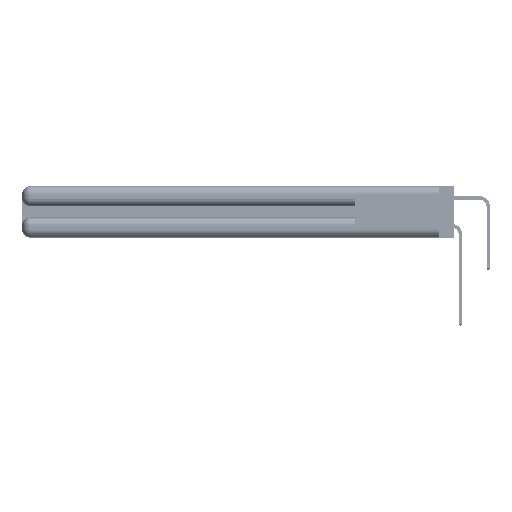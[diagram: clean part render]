
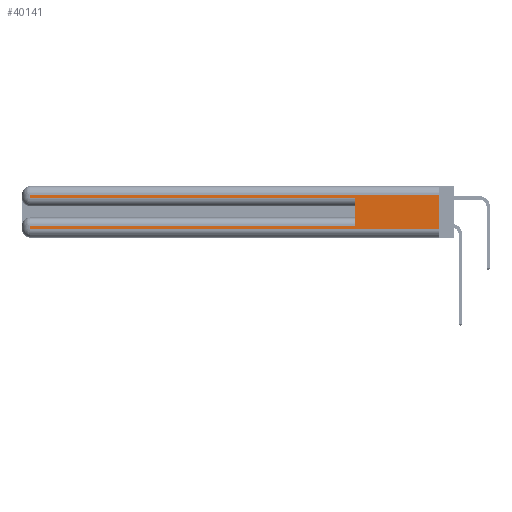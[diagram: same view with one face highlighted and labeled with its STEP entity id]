
A CAD part, left-side view. The second image highlights one B-rep face of the part: STEP entity #40141.
In plain terms, the highlighted planar face has unit normal (-1, 0, 0).
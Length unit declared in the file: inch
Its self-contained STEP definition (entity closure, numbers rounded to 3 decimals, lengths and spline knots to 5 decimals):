
#798 = VERTEX_POINT ( 'NONE', #17650 ) ;
#2021 = CARTESIAN_POINT ( 'NONE',  ( 0., 2.94, 0.06 ) ) ;
#2436 = ORIENTED_EDGE ( 'NONE', *, *, #35362, .T. ) ;
#2768 = CARTESIAN_POINT ( 'NONE',  ( 0., 2.94, 0.285 ) ) ;
#2984 = EDGE_CURVE ( 'NONE', #15669, #55443, #12551, .T. ) ;
#4035 = EDGE_CURVE ( 'NONE', #9120, #798, #41497, .T. ) ;
#4609 = CARTESIAN_POINT ( 'NONE',  ( 0., 2.94, 0.31 ) ) ;
#4824 = VERTEX_POINT ( 'NONE', #26628 ) ;
#4967 = ORIENTED_EDGE ( 'NONE', *, *, #2984, .F. ) ;
#5158 = CARTESIAN_POINT ( 'NONE',  ( 0., 0., 0.085 ) ) ;
#5236 = EDGE_CURVE ( 'NONE', #55634, #798, #55422, .T. ) ;
#5494 = LINE ( 'NONE', #29674, #10962 ) ;
#9120 = VERTEX_POINT ( 'NONE', #2021 ) ;
#10962 = VECTOR ( 'NONE', #12107, 39.37008 ) ;
#11747 = ORIENTED_EDGE ( 'NONE', *, *, #28604, .T. ) ;
#12107 = DIRECTION ( 'NONE',  ( 0., 1., 0. ) ) ;
#12335 = LINE ( 'NONE', #5158, #55706 ) ;
#12377 = DIRECTION ( 'NONE',  ( 1., 0., 0. ) ) ;
#12551 = LINE ( 'NONE', #27967, #22717 ) ;
#12958 = DIRECTION ( 'NONE',  ( 0., -1., 0. ) ) ;
#13211 = DIRECTION ( 'NONE',  ( 0., 0., -1. ) ) ;
#14215 = LINE ( 'NONE', #51944, #25746 ) ;
#14616 = CARTESIAN_POINT ( 'NONE',  ( 0., 0., 0.31 ) ) ;
#15669 = VERTEX_POINT ( 'NONE', #37559 ) ;
#16627 = FACE_OUTER_BOUND ( 'NONE', #29875, .T. ) ;
#16932 = CARTESIAN_POINT ( 'NONE',  ( 0., 0., 0.37 ) ) ;
#17650 = CARTESIAN_POINT ( 'NONE',  ( 0., 0., 0.06 ) ) ;
#20690 = CARTESIAN_POINT ( 'NONE',  ( 0., 0., 0.37 ) ) ;
#21822 = AXIS2_PLACEMENT_3D ( 'NONE', #16932, #12377, #33522 ) ;
#22451 = DIRECTION ( 'NONE',  ( 0., 1., 0. ) ) ;
#22717 = VECTOR ( 'NONE', #36632, 39.37008 ) ;
#23726 = CARTESIAN_POINT ( 'NONE',  ( 0., 0.6, 0.285 ) ) ;
#24527 = EDGE_CURVE ( 'NONE', #15669, #4824, #12335, .T. ) ;
#24696 = EDGE_CURVE ( 'NONE', #55634, #25555, #5494, .T. ) ;
#24818 = VECTOR ( 'NONE', #53105, 39.37008 ) ;
#25555 = VERTEX_POINT ( 'NONE', #4609 ) ;
#25746 = VECTOR ( 'NONE', #12958, 39.37008 ) ;
#26230 = ORIENTED_EDGE ( 'NONE', *, *, #5236, .F. ) ;
#26628 = CARTESIAN_POINT ( 'NONE',  ( 0., 2.94, 0.085 ) ) ;
#27967 = CARTESIAN_POINT ( 'NONE',  ( 0., 0.6, 0.145 ) ) ;
#28604 = EDGE_CURVE ( 'NONE', #25555, #34652, #41723, .T. ) ;
#28907 = VECTOR ( 'NONE', #13211, 39.37008 ) ;
#29674 = CARTESIAN_POINT ( 'NONE',  ( 0., 0., 0.31 ) ) ;
#29875 = EDGE_LOOP ( 'NONE', ( #26230, #30563, #11747, #2436, #4967, #53065, #35982, #38648 ) ) ;
#30563 = ORIENTED_EDGE ( 'NONE', *, *, #24696, .T. ) ;
#30599 = CARTESIAN_POINT ( 'NONE',  ( 0., 2.94, 0.37 ) ) ;
#31570 = EDGE_CURVE ( 'NONE', #4824, #9120, #37678, .T. ) ;
#33522 = DIRECTION ( 'NONE',  ( 0., 0., -1. ) ) ;
#34652 = VERTEX_POINT ( 'NONE', #2768 ) ;
#35362 = EDGE_CURVE ( 'NONE', #34652, #55443, #14215, .T. ) ;
#35982 = ORIENTED_EDGE ( 'NONE', *, *, #31570, .T. ) ;
#36632 = DIRECTION ( 'NONE',  ( 0., 0., 1. ) ) ;
#37559 = CARTESIAN_POINT ( 'NONE',  ( 0., 0.6, 0.085 ) ) ;
#37678 = LINE ( 'NONE', #30599, #28907 ) ;
#38648 = ORIENTED_EDGE ( 'NONE', *, *, #4035, .T. ) ;
#39774 = CARTESIAN_POINT ( 'NONE',  ( 0., 2.94, 0.37 ) ) ;
#40141 = ADVANCED_FACE ( 'NONE', ( #16627 ), #47186, .F. ) ;
#41497 = LINE ( 'NONE', #44248, #42888 ) ;
#41723 = LINE ( 'NONE', #39774, #24818 ) ;
#42888 = VECTOR ( 'NONE', #43868, 39.37008 ) ;
#43858 = VECTOR ( 'NONE', #50975, 39.37008 ) ;
#43868 = DIRECTION ( 'NONE',  ( 0., -1., 0. ) ) ;
#44248 = CARTESIAN_POINT ( 'NONE',  ( 0., 0., 0.06 ) ) ;
#47186 = PLANE ( 'NONE',  #21822 ) ;
#50975 = DIRECTION ( 'NONE',  ( 0., 0., -1. ) ) ;
#51944 = CARTESIAN_POINT ( 'NONE',  ( 0., 0., 0.285 ) ) ;
#53065 = ORIENTED_EDGE ( 'NONE', *, *, #24527, .T. ) ;
#53105 = DIRECTION ( 'NONE',  ( 0., 0., -1. ) ) ;
#55422 = LINE ( 'NONE', #20690, #43858 ) ;
#55443 = VERTEX_POINT ( 'NONE', #23726 ) ;
#55634 = VERTEX_POINT ( 'NONE', #14616 ) ;
#55706 = VECTOR ( 'NONE', #22451, 39.37008 ) ;
